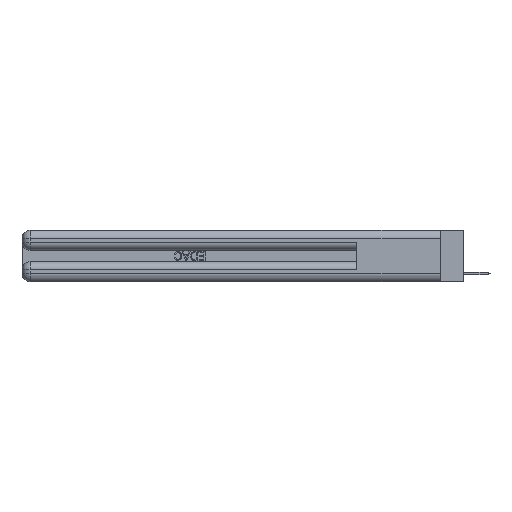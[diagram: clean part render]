
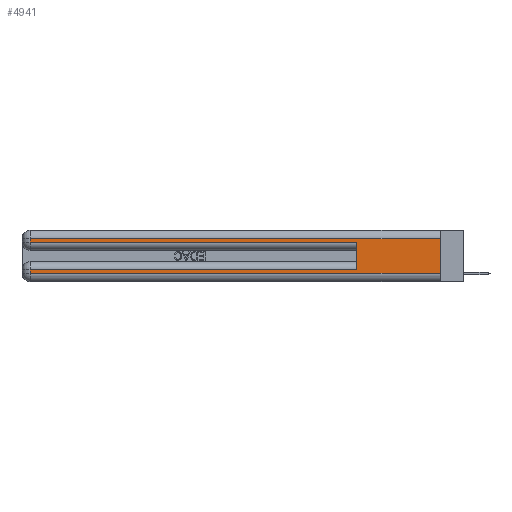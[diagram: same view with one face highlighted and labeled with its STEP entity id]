
A CAD part, left-side view. The second image highlights one B-rep face of the part: STEP entity #4941.
In plain terms, the highlighted planar face has unit normal (-1, 0, 0).
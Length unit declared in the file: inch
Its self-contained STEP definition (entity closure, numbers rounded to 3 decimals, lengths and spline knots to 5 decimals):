
#67 = CARTESIAN_POINT ( 'NONE',  ( 0., 0., 0.31 ) ) ;
#641 = VERTEX_POINT ( 'NONE', #16293 ) ;
#947 = CARTESIAN_POINT ( 'NONE',  ( 0., 2.94, 0.37 ) ) ;
#981 = VERTEX_POINT ( 'NONE', #23230 ) ;
#1027 = CARTESIAN_POINT ( 'NONE',  ( 0., 0., 0.37 ) ) ;
#1309 = PLANE ( 'NONE',  #8507 ) ;
#1331 = LINE ( 'NONE', #10133, #21023 ) ;
#1553 = CARTESIAN_POINT ( 'NONE',  ( 0., 0., 0.06 ) ) ;
#1909 = EDGE_CURVE ( 'NONE', #14748, #14247, #1331, .T. ) ;
#2122 = VECTOR ( 'NONE', #25773, 39.37008 ) ;
#2207 = CARTESIAN_POINT ( 'NONE',  ( 0., 0., 0.085 ) ) ;
#2240 = VERTEX_POINT ( 'NONE', #13222 ) ;
#2603 = VERTEX_POINT ( 'NONE', #23922 ) ;
#3188 = ORIENTED_EDGE ( 'NONE', *, *, #22523, .T. ) ;
#3321 = DIRECTION ( 'NONE',  ( 1., 0., 0. ) ) ;
#3454 = VERTEX_POINT ( 'NONE', #14851 ) ;
#3536 = EDGE_CURVE ( 'NONE', #981, #2603, #17466, .T. ) ;
#3984 = EDGE_CURVE ( 'NONE', #14748, #26837, #14231, .T. ) ;
#4026 = LINE ( 'NONE', #14849, #17620 ) ;
#4941 = ADVANCED_FACE ( 'NONE', ( #18919 ), #1309, .F. ) ;
#5853 = CARTESIAN_POINT ( 'NONE',  ( 0., 0., 0.31 ) ) ;
#5914 = EDGE_CURVE ( 'NONE', #641, #2603, #8120, .T. ) ;
#6530 = VECTOR ( 'NONE', #20481, 39.37008 ) ;
#8120 = LINE ( 'NONE', #16938, #2122 ) ;
#8429 = ORIENTED_EDGE ( 'NONE', *, *, #3984, .T. ) ;
#8507 = AXIS2_PLACEMENT_3D ( 'NONE', #1027, #3321, #9826 ) ;
#9417 = VECTOR ( 'NONE', #15568, 39.37008 ) ;
#9745 = DIRECTION ( 'NONE',  ( 0., 0., -1. ) ) ;
#9826 = DIRECTION ( 'NONE',  ( 0., 0., -1. ) ) ;
#10133 = CARTESIAN_POINT ( 'NONE',  ( 0., 0., 0.37 ) ) ;
#10435 = VECTOR ( 'NONE', #11009, 39.37008 ) ;
#10603 = ORIENTED_EDGE ( 'NONE', *, *, #1909, .F. ) ;
#11009 = DIRECTION ( 'NONE',  ( 0., 1., 0. ) ) ;
#11178 = EDGE_CURVE ( 'NONE', #981, #2240, #19389, .T. ) ;
#11253 = ORIENTED_EDGE ( 'NONE', *, *, #5914, .T. ) ;
#11905 = LINE ( 'NONE', #947, #26425 ) ;
#13222 = CARTESIAN_POINT ( 'NONE',  ( 0., 2.94, 0.085 ) ) ;
#13962 = LINE ( 'NONE', #22522, #6530 ) ;
#14231 = LINE ( 'NONE', #5853, #19082 ) ;
#14247 = VERTEX_POINT ( 'NONE', #1553 ) ;
#14748 = VERTEX_POINT ( 'NONE', #67 ) ;
#14849 = CARTESIAN_POINT ( 'NONE',  ( 0., 2.94, 0.37 ) ) ;
#14851 = CARTESIAN_POINT ( 'NONE',  ( 0., 2.94, 0.06 ) ) ;
#15174 = ORIENTED_EDGE ( 'NONE', *, *, #11178, .T. ) ;
#15568 = DIRECTION ( 'NONE',  ( 0., 0., 1. ) ) ;
#15711 = CARTESIAN_POINT ( 'NONE',  ( 0., 0.6, 0.145 ) ) ;
#15961 = ORIENTED_EDGE ( 'NONE', *, *, #21794, .T. ) ;
#16293 = CARTESIAN_POINT ( 'NONE',  ( 0., 2.94, 0.285 ) ) ;
#16938 = CARTESIAN_POINT ( 'NONE',  ( 0., 0., 0.285 ) ) ;
#17466 = LINE ( 'NONE', #15711, #9417 ) ;
#17620 = VECTOR ( 'NONE', #28459, 39.37008 ) ;
#18919 = FACE_OUTER_BOUND ( 'NONE', #24575, .T. ) ;
#18936 = DIRECTION ( 'NONE',  ( 0., 0., -1. ) ) ;
#19082 = VECTOR ( 'NONE', #27538, 39.37008 ) ;
#19389 = LINE ( 'NONE', #2207, #10435 ) ;
#20481 = DIRECTION ( 'NONE',  ( 0., -1., 0. ) ) ;
#21023 = VECTOR ( 'NONE', #18936, 39.37008 ) ;
#21794 = EDGE_CURVE ( 'NONE', #26837, #641, #4026, .T. ) ;
#22522 = CARTESIAN_POINT ( 'NONE',  ( 0., 0., 0.06 ) ) ;
#22523 = EDGE_CURVE ( 'NONE', #2240, #3454, #11905, .T. ) ;
#23170 = EDGE_CURVE ( 'NONE', #3454, #14247, #13962, .T. ) ;
#23230 = CARTESIAN_POINT ( 'NONE',  ( 0., 0.6, 0.085 ) ) ;
#23922 = CARTESIAN_POINT ( 'NONE',  ( 0., 0.6, 0.285 ) ) ;
#24017 = ORIENTED_EDGE ( 'NONE', *, *, #3536, .F. ) ;
#24575 = EDGE_LOOP ( 'NONE', ( #10603, #8429, #15961, #11253, #24017, #15174, #3188, #25294 ) ) ;
#25294 = ORIENTED_EDGE ( 'NONE', *, *, #23170, .T. ) ;
#25773 = DIRECTION ( 'NONE',  ( 0., -1., 0. ) ) ;
#26425 = VECTOR ( 'NONE', #9745, 39.37008 ) ;
#26837 = VERTEX_POINT ( 'NONE', #26858 ) ;
#26858 = CARTESIAN_POINT ( 'NONE',  ( 0., 2.94, 0.31 ) ) ;
#27538 = DIRECTION ( 'NONE',  ( 0., 1., 0. ) ) ;
#28459 = DIRECTION ( 'NONE',  ( 0., 0., -1. ) ) ;
